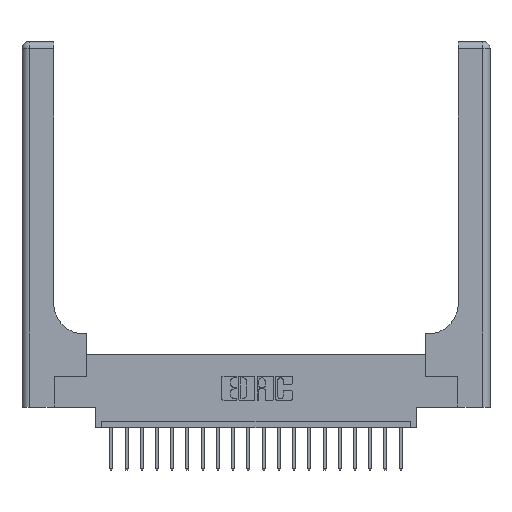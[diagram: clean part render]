
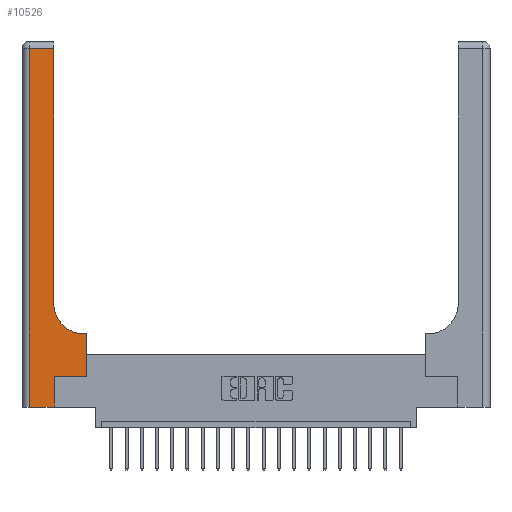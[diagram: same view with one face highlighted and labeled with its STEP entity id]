
A CAD part, top view. The second image highlights one B-rep face of the part: STEP entity #10526.
In plain terms, the highlighted planar face has unit normal (0, 0, 1).
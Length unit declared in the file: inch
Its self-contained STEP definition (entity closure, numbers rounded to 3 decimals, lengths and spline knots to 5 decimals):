
#355 = ORIENTED_EDGE ( 'NONE', *, *, #11695, .T. ) ;
#451 = DIRECTION ( 'NONE',  ( 0., 1., 0. ) ) ;
#1112 = CARTESIAN_POINT ( 'NONE',  ( 0.528, 0.6, 0.37 ) ) ;
#1122 = EDGE_CURVE ( 'NONE', #8362, #2790, #12892, .T. ) ;
#1128 = CARTESIAN_POINT ( 'NONE',  ( 0.06, 3., 0.37 ) ) ;
#1810 = LINE ( 'NONE', #9725, #4245 ) ;
#2104 = ORIENTED_EDGE ( 'NONE', *, *, #14417, .T. ) ;
#2674 = VERTEX_POINT ( 'NONE', #1112 ) ;
#2790 = VERTEX_POINT ( 'NONE', #12654 ) ;
#3020 = EDGE_CURVE ( 'NONE', #15310, #8362, #6956, .T. ) ;
#3416 = CARTESIAN_POINT ( 'NONE',  ( 0.265, 0.25, 0.37 ) ) ;
#4245 = VECTOR ( 'NONE', #19562, 39.37008 ) ;
#4612 = CIRCLE ( 'NONE', #13845, 0.25 ) ;
#4708 = EDGE_CURVE ( 'NONE', #14600, #15310, #4612, .T. ) ;
#4725 = VERTEX_POINT ( 'NONE', #3416 ) ;
#4919 = CARTESIAN_POINT ( 'NONE',  ( 0.265, 0.25, 0.37 ) ) ;
#4920 = DIRECTION ( 'NONE',  ( 1., 0., 0. ) ) ;
#5205 = CARTESIAN_POINT ( 'NONE',  ( 0.26, 2.94, 0.37 ) ) ;
#5931 = LINE ( 'NONE', #11067, #16565 ) ;
#6037 = DIRECTION ( 'NONE',  ( -1., 0., 0. ) ) ;
#6133 = DIRECTION ( 'NONE',  ( -1., 0., 0. ) ) ;
#6280 = CARTESIAN_POINT ( 'NONE',  ( 0.265, 0., 0.37 ) ) ;
#6519 = LINE ( 'NONE', #4919, #20369 ) ;
#6956 = LINE ( 'NONE', #15086, #11642 ) ;
#7348 = ORIENTED_EDGE ( 'NONE', *, *, #10142, .T. ) ;
#7523 = PLANE ( 'NONE',  #13987 ) ;
#7630 = CARTESIAN_POINT ( 'NONE',  ( 0.06, 0., 0.37 ) ) ;
#8362 = VERTEX_POINT ( 'NONE', #5205 ) ;
#8645 = VERTEX_POINT ( 'NONE', #15635 ) ;
#9061 = ORIENTED_EDGE ( 'NONE', *, *, #15719, .T. ) ;
#9415 = DIRECTION ( 'NONE',  ( 1., 0., 0. ) ) ;
#9725 = CARTESIAN_POINT ( 'NONE',  ( 0., 0., 0.37 ) ) ;
#10142 = EDGE_CURVE ( 'NONE', #8645, #2674, #10661, .T. ) ;
#10526 = ADVANCED_FACE ( 'NONE', ( #20796 ), #7523, .F. ) ;
#10661 = LINE ( 'NONE', #20823, #10938 ) ;
#10741 = CARTESIAN_POINT ( 'NONE',  ( 0., 3., 0.37 ) ) ;
#10865 = ORIENTED_EDGE ( 'NONE', *, *, #3020, .T. ) ;
#10938 = VECTOR ( 'NONE', #13981, 39.37008 ) ;
#11067 = CARTESIAN_POINT ( 'NONE',  ( 0.26, 0.6, 0.37 ) ) ;
#11169 = ORIENTED_EDGE ( 'NONE', *, *, #18666, .T. ) ;
#11642 = VECTOR ( 'NONE', #451, 39.37008 ) ;
#11695 = EDGE_CURVE ( 'NONE', #2790, #11700, #15564, .T. ) ;
#11700 = VERTEX_POINT ( 'NONE', #7630 ) ;
#12654 = CARTESIAN_POINT ( 'NONE',  ( 0.06, 2.94, 0.37 ) ) ;
#12892 = LINE ( 'NONE', #14271, #14576 ) ;
#13569 = DIRECTION ( 'NONE',  ( 0., 0., -1. ) ) ;
#13630 = ORIENTED_EDGE ( 'NONE', *, *, #20180, .T. ) ;
#13845 = AXIS2_PLACEMENT_3D ( 'NONE', #19991, #13569, #4920 ) ;
#13956 = DIRECTION ( 'NONE',  ( -1., 0., 0. ) ) ;
#13981 = DIRECTION ( 'NONE',  ( 0., 1., 0. ) ) ;
#13987 = AXIS2_PLACEMENT_3D ( 'NONE', #10741, #14263, #13956 ) ;
#14231 = ORIENTED_EDGE ( 'NONE', *, *, #1122, .T. ) ;
#14263 = DIRECTION ( 'NONE',  ( 0., 0., -1. ) ) ;
#14271 = CARTESIAN_POINT ( 'NONE',  ( 0., 2.94, 0.37 ) ) ;
#14360 = VECTOR ( 'NONE', #15971, 39.37008 ) ;
#14417 = EDGE_CURVE ( 'NONE', #20695, #4725, #18833, .T. ) ;
#14464 = EDGE_LOOP ( 'NONE', ( #10865, #14231, #355, #9061, #2104, #13630, #7348, #11169, #18628 ) ) ;
#14576 = VECTOR ( 'NONE', #6133, 39.37008 ) ;
#14600 = VERTEX_POINT ( 'NONE', #14825 ) ;
#14825 = CARTESIAN_POINT ( 'NONE',  ( 0.51, 0.6, 0.37 ) ) ;
#15086 = CARTESIAN_POINT ( 'NONE',  ( 0.26, 3., 0.37 ) ) ;
#15310 = VERTEX_POINT ( 'NONE', #17777 ) ;
#15564 = LINE ( 'NONE', #1128, #14360 ) ;
#15635 = CARTESIAN_POINT ( 'NONE',  ( 0.528, 0.25, 0.37 ) ) ;
#15719 = EDGE_CURVE ( 'NONE', #11700, #20695, #1810, .T. ) ;
#15971 = DIRECTION ( 'NONE',  ( 0., -1., 0. ) ) ;
#16565 = VECTOR ( 'NONE', #6037, 39.37008 ) ;
#17777 = CARTESIAN_POINT ( 'NONE',  ( 0.26, 0.85, 0.37 ) ) ;
#18628 = ORIENTED_EDGE ( 'NONE', *, *, #4708, .T. ) ;
#18666 = EDGE_CURVE ( 'NONE', #2674, #14600, #5931, .T. ) ;
#18833 = LINE ( 'NONE', #6280, #20609 ) ;
#19562 = DIRECTION ( 'NONE',  ( 1., 0., 0. ) ) ;
#19991 = CARTESIAN_POINT ( 'NONE',  ( 0.51, 0.85, 0.37 ) ) ;
#20180 = EDGE_CURVE ( 'NONE', #4725, #8645, #6519, .T. ) ;
#20369 = VECTOR ( 'NONE', #9415, 39.37008 ) ;
#20370 = CARTESIAN_POINT ( 'NONE',  ( 0.265, 0., 0.37 ) ) ;
#20609 = VECTOR ( 'NONE', #21048, 39.37008 ) ;
#20695 = VERTEX_POINT ( 'NONE', #20370 ) ;
#20796 = FACE_OUTER_BOUND ( 'NONE', #14464, .T. ) ;
#20823 = CARTESIAN_POINT ( 'NONE',  ( 0.528, 0.25, 0.37 ) ) ;
#21048 = DIRECTION ( 'NONE',  ( 0., 1., 0. ) ) ;
